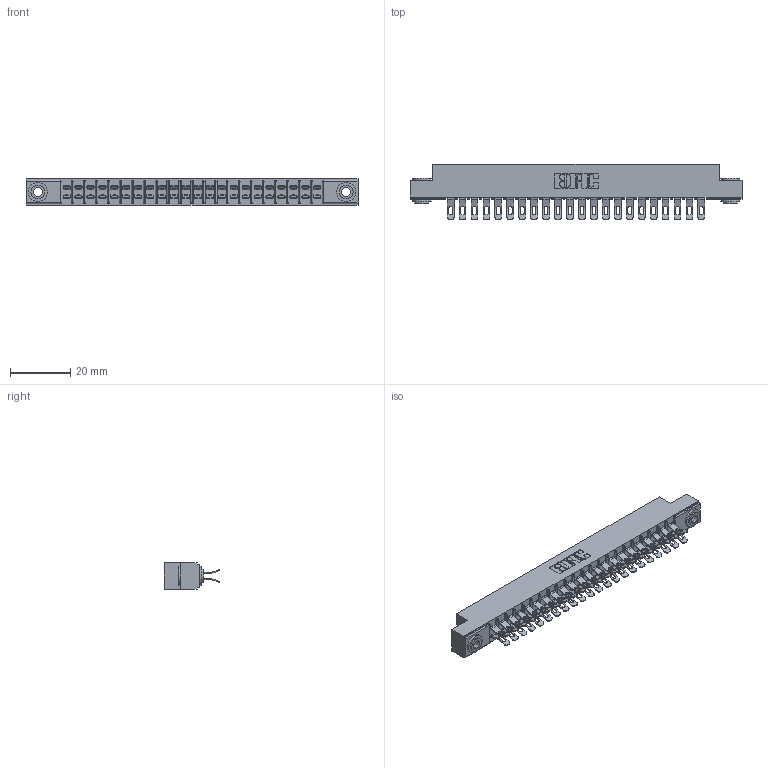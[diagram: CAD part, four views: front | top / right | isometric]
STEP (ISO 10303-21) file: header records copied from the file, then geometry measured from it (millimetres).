
FILE_DESCRIPTION (( 'STEP AP203' ), '1' );
FILE_NAME ('355-044-555-203.STEP', '2019-09-11T14:17:37', ( '' ), ( '' ), 'SwSTEP 2.0', 'SolidWorks 2016', '' );
FILE_SCHEMA (( 'CONFIG_CONTROL_DESIGN' ));
Length unit declared in the file: inch
Products named in the file (4): 305-290-001_555; 345-250-002_345-250-002-102; 305 Part_.156 Dia; 355-044-555-203
Assembly tree (47 placements, depth 2):
  355-044-555-203
    305 Part_.156 Dia
    305-290-001_555  x44
    345-250-002_345-250-002-102  x2
Bounding box: 110.19 x 18.41 x 8.71 mm (x, y, z)
Volume: 7037.7 mm3; surface area: 14294 mm2
Topology: 47 solids, 47 shells, 3072 faces, 9118 edges, 5956 vertices
Faces by surface type: plane 1500, cylinder 1476, sphere 88, cone 8
Entity records: 27944 total; most frequent: CARTESIAN_POINT 4623, ORIENTED_EDGE 4568, DIRECTION 4498, EDGE_CURVE 2284, LINE 1796, VECTOR 1796, VERTEX_POINT 1460, AXIS2_PLACEMENT_3D 1351
